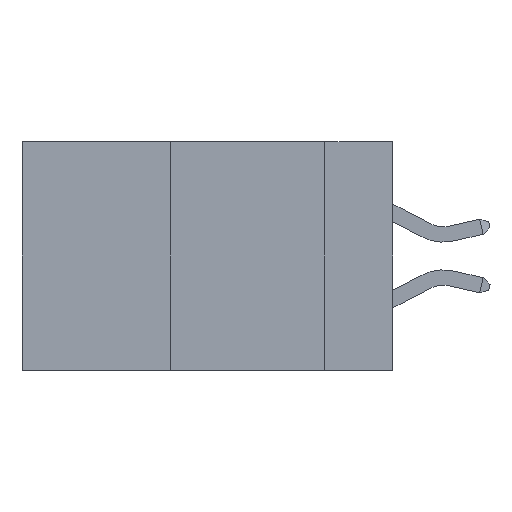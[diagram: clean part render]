
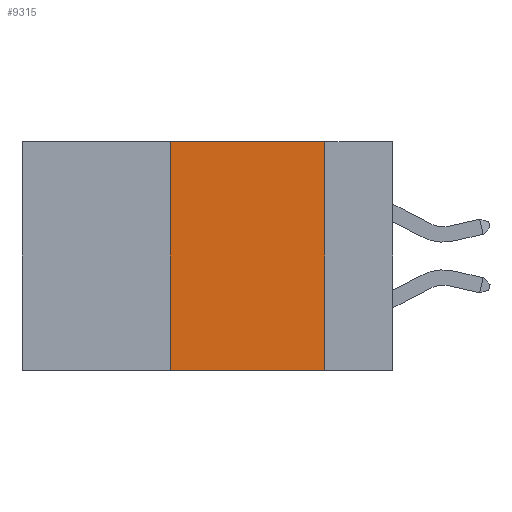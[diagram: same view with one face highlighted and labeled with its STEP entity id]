
A CAD part, left-side view. The second image highlights one B-rep face of the part: STEP entity #9315.
In plain terms, the highlighted planar face has unit normal (-1, 0, 0).
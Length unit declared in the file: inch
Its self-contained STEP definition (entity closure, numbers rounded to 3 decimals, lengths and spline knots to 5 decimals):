
#175 = ORIENTED_EDGE ( 'NONE', *, *, #2030, .T. ) ;
#309 = LINE ( 'NONE', #3677, #1298 ) ;
#557 = DIRECTION ( 'NONE',  ( 0., 0., -1. ) ) ;
#996 = CARTESIAN_POINT ( 'NONE',  ( 0., 0.36, -0.37 ) ) ;
#1298 = VECTOR ( 'NONE', #2773, 39.37008 ) ;
#1535 = LINE ( 'NONE', #4109, #3797 ) ;
#1666 = CARTESIAN_POINT ( 'NONE',  ( 0., 0.11, 0. ) ) ;
#1943 = VERTEX_POINT ( 'NONE', #6723 ) ;
#2030 = EDGE_CURVE ( 'NONE', #6747, #11554, #4299, .T. ) ;
#2115 = EDGE_CURVE ( 'NONE', #6747, #1943, #309, .T. ) ;
#2376 = PLANE ( 'NONE',  #6444 ) ;
#2773 = DIRECTION ( 'NONE',  ( 0., 0., 1. ) ) ;
#3677 = CARTESIAN_POINT ( 'NONE',  ( 0., 0.36, 0. ) ) ;
#3797 = VECTOR ( 'NONE', #557, 39.37008 ) ;
#3908 = CARTESIAN_POINT ( 'NONE',  ( 0., 0.11, -0.37 ) ) ;
#4109 = CARTESIAN_POINT ( 'NONE',  ( 0., 0.11, 0. ) ) ;
#4299 = LINE ( 'NONE', #7936, #6419 ) ;
#5135 = CARTESIAN_POINT ( 'NONE',  ( 0., 0.6, 0. ) ) ;
#5799 = FACE_OUTER_BOUND ( 'NONE', #11659, .T. ) ;
#6419 = VECTOR ( 'NONE', #10715, 39.37008 ) ;
#6444 = AXIS2_PLACEMENT_3D ( 'NONE', #6924, #8886, #7922 ) ;
#6723 = CARTESIAN_POINT ( 'NONE',  ( 0., 0.36, 0. ) ) ;
#6747 = VERTEX_POINT ( 'NONE', #996 ) ;
#6924 = CARTESIAN_POINT ( 'NONE',  ( 0., 0.6, 0. ) ) ;
#7417 = ORIENTED_EDGE ( 'NONE', *, *, #2115, .F. ) ;
#7827 = DIRECTION ( 'NONE',  ( 0., -1., 0. ) ) ;
#7922 = DIRECTION ( 'NONE',  ( 0., 0., -1. ) ) ;
#7936 = CARTESIAN_POINT ( 'NONE',  ( 0., 0.6, -0.37 ) ) ;
#8009 = EDGE_CURVE ( 'NONE', #1943, #9952, #10193, .T. ) ;
#8709 = ORIENTED_EDGE ( 'NONE', *, *, #8802, .F. ) ;
#8802 = EDGE_CURVE ( 'NONE', #9952, #11554, #1535, .T. ) ;
#8886 = DIRECTION ( 'NONE',  ( 1., 0., 0. ) ) ;
#9291 = ORIENTED_EDGE ( 'NONE', *, *, #8009, .F. ) ;
#9315 = ADVANCED_FACE ( 'NONE', ( #5799 ), #2376, .F. ) ;
#9952 = VERTEX_POINT ( 'NONE', #1666 ) ;
#10193 = LINE ( 'NONE', #5135, #10336 ) ;
#10336 = VECTOR ( 'NONE', #7827, 39.37008 ) ;
#10715 = DIRECTION ( 'NONE',  ( 0., -1., 0. ) ) ;
#11554 = VERTEX_POINT ( 'NONE', #3908 ) ;
#11659 = EDGE_LOOP ( 'NONE', ( #8709, #9291, #7417, #175 ) ) ;
